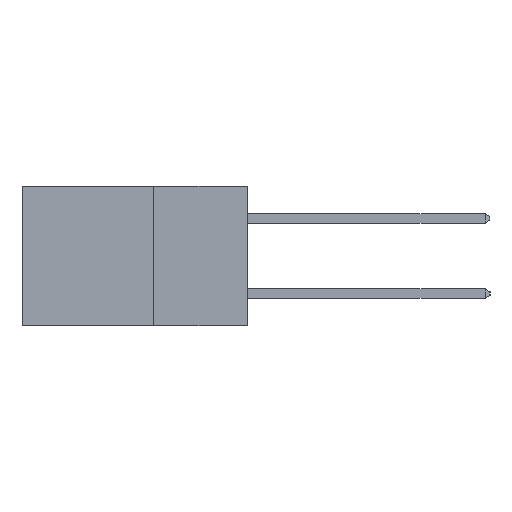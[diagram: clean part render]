
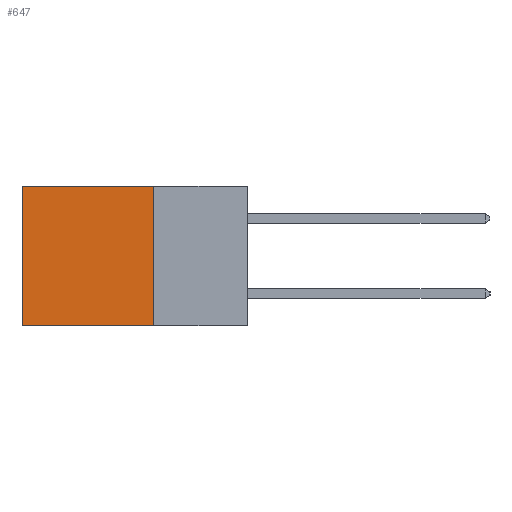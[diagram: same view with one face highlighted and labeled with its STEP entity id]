
A CAD part, left-side view. The second image highlights one B-rep face of the part: STEP entity #647.
In plain terms, the highlighted planar face has unit normal (-1, 0, 0).
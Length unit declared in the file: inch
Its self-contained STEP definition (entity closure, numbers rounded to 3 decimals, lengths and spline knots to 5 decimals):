
#616 = ORIENTED_EDGE ( 'NONE', *, *, #2582, .T. ) ;
#647 = ADVANCED_FACE ( 'NONE', ( #2923 ), #14568, .F. ) ;
#927 = DIRECTION ( 'NONE',  ( 0., 0., -1. ) ) ;
#1917 = DIRECTION ( 'NONE',  ( 0., 0., -1. ) ) ;
#2014 = VERTEX_POINT ( 'NONE', #2877 ) ;
#2301 = VERTEX_POINT ( 'NONE', #12346 ) ;
#2582 = EDGE_CURVE ( 'NONE', #8091, #2014, #3426, .T. ) ;
#2851 = CARTESIAN_POINT ( 'NONE',  ( 0.2615, 0.25, -0.37 ) ) ;
#2877 = CARTESIAN_POINT ( 'NONE',  ( 0.2615, 0.6, 0. ) ) ;
#2923 = FACE_OUTER_BOUND ( 'NONE', #13470, .T. ) ;
#3426 = LINE ( 'NONE', #4229, #12434 ) ;
#3882 = DIRECTION ( 'NONE',  ( 0., 1., 0. ) ) ;
#4229 = CARTESIAN_POINT ( 'NONE',  ( 0.2615, 0.25, 0. ) ) ;
#4425 = ORIENTED_EDGE ( 'NONE', *, *, #8889, .T. ) ;
#4614 = ORIENTED_EDGE ( 'NONE', *, *, #10777, .F. ) ;
#4698 = VECTOR ( 'NONE', #1917, 39.37008 ) ;
#5060 = VECTOR ( 'NONE', #6353, 39.37008 ) ;
#5350 = CARTESIAN_POINT ( 'NONE',  ( 0.2615, 0.25, 0. ) ) ;
#6066 = ORIENTED_EDGE ( 'NONE', *, *, #9670, .F. ) ;
#6353 = DIRECTION ( 'NONE',  ( 0., 1., 0. ) ) ;
#7482 = LINE ( 'NONE', #10686, #4698 ) ;
#7527 = DIRECTION ( 'NONE',  ( 0., 0., -1. ) ) ;
#7560 = CARTESIAN_POINT ( 'NONE',  ( 0.2615, 0.25, -0.37 ) ) ;
#7679 = DIRECTION ( 'NONE',  ( 1., 0., 0. ) ) ;
#8087 = VECTOR ( 'NONE', #927, 39.37008 ) ;
#8091 = VERTEX_POINT ( 'NONE', #5350 ) ;
#8142 = CARTESIAN_POINT ( 'NONE',  ( 0.2615, 0.25, -0.37 ) ) ;
#8889 = EDGE_CURVE ( 'NONE', #2014, #10821, #7482, .T. ) ;
#8914 = CARTESIAN_POINT ( 'NONE',  ( 0.2615, 0.6, -0.37 ) ) ;
#9670 = EDGE_CURVE ( 'NONE', #8091, #2301, #10835, .T. ) ;
#10390 = AXIS2_PLACEMENT_3D ( 'NONE', #7560, #7679, #7527 ) ;
#10686 = CARTESIAN_POINT ( 'NONE',  ( 0.2615, 0.6, -0.37 ) ) ;
#10777 = EDGE_CURVE ( 'NONE', #2301, #10821, #14002, .T. ) ;
#10821 = VERTEX_POINT ( 'NONE', #8914 ) ;
#10835 = LINE ( 'NONE', #8142, #8087 ) ;
#12346 = CARTESIAN_POINT ( 'NONE',  ( 0.2615, 0.25, -0.37 ) ) ;
#12434 = VECTOR ( 'NONE', #3882, 39.37008 ) ;
#13470 = EDGE_LOOP ( 'NONE', ( #4425, #4614, #6066, #616 ) ) ;
#14002 = LINE ( 'NONE', #2851, #5060 ) ;
#14568 = PLANE ( 'NONE',  #10390 ) ;
